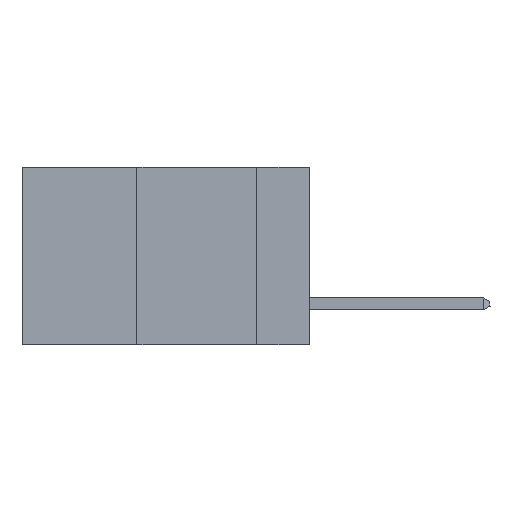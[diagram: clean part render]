
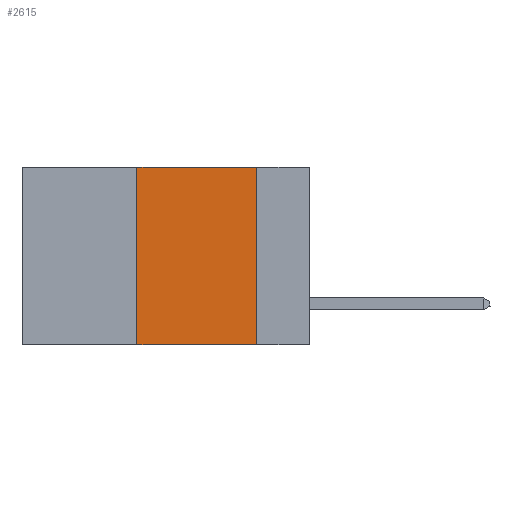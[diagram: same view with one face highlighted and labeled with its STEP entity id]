
A CAD part, left-side view. The second image highlights one B-rep face of the part: STEP entity #2615.
In plain terms, the highlighted planar face has unit normal (-1, 0, 0).
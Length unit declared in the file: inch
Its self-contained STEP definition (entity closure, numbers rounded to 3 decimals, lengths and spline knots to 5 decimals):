
#247 = CARTESIAN_POINT ( 'NONE',  ( 0., 0.11, -0.37 ) ) ;
#796 = CARTESIAN_POINT ( 'NONE',  ( 0., 0.6, 0. ) ) ;
#1013 = VECTOR ( 'NONE', #9403, 39.37008 ) ;
#1615 = EDGE_CURVE ( 'NONE', #12031, #11859, #6972, .T. ) ;
#2241 = DIRECTION ( 'NONE',  ( 0., 0., -1. ) ) ;
#2468 = AXIS2_PLACEMENT_3D ( 'NONE', #796, #4886, #2241 ) ;
#2615 = ADVANCED_FACE ( 'NONE', ( #13251 ), #14352, .F. ) ;
#3099 = LINE ( 'NONE', #13943, #3928 ) ;
#3928 = VECTOR ( 'NONE', #15187, 39.37008 ) ;
#4886 = DIRECTION ( 'NONE',  ( 1., 0., 0. ) ) ;
#5456 = VERTEX_POINT ( 'NONE', #12373 ) ;
#5460 = EDGE_CURVE ( 'NONE', #12031, #5456, #16967, .T. ) ;
#6972 = LINE ( 'NONE', #14789, #1013 ) ;
#7619 = ORIENTED_EDGE ( 'NONE', *, *, #5460, .F. ) ;
#8349 = CARTESIAN_POINT ( 'NONE',  ( 0., 0.36, 0. ) ) ;
#9403 = DIRECTION ( 'NONE',  ( 0., -1., 0. ) ) ;
#10386 = CARTESIAN_POINT ( 'NONE',  ( 0., 0.36, -0.37 ) ) ;
#10608 = VECTOR ( 'NONE', #14988, 39.37008 ) ;
#11859 = VERTEX_POINT ( 'NONE', #247 ) ;
#12031 = VERTEX_POINT ( 'NONE', #10386 ) ;
#12373 = CARTESIAN_POINT ( 'NONE',  ( 0., 0.36, 0. ) ) ;
#13206 = ORIENTED_EDGE ( 'NONE', *, *, #1615, .T. ) ;
#13251 = FACE_OUTER_BOUND ( 'NONE', #14702, .T. ) ;
#13943 = CARTESIAN_POINT ( 'NONE',  ( 0., 0.11, 0. ) ) ;
#14039 = ORIENTED_EDGE ( 'NONE', *, *, #15873, .F. ) ;
#14069 = CARTESIAN_POINT ( 'NONE',  ( 0., 0.6, 0. ) ) ;
#14299 = DIRECTION ( 'NONE',  ( 0., -1., 0. ) ) ;
#14352 = PLANE ( 'NONE',  #2468 ) ;
#14528 = LINE ( 'NONE', #14069, #16883 ) ;
#14702 = EDGE_LOOP ( 'NONE', ( #14039, #16604, #7619, #13206 ) ) ;
#14789 = CARTESIAN_POINT ( 'NONE',  ( 0., 0.6, -0.37 ) ) ;
#14988 = DIRECTION ( 'NONE',  ( 0., 0., 1. ) ) ;
#15106 = CARTESIAN_POINT ( 'NONE',  ( 0., 0.11, 0. ) ) ;
#15187 = DIRECTION ( 'NONE',  ( 0., 0., -1. ) ) ;
#15440 = EDGE_CURVE ( 'NONE', #5456, #16450, #14528, .T. ) ;
#15873 = EDGE_CURVE ( 'NONE', #16450, #11859, #3099, .T. ) ;
#16450 = VERTEX_POINT ( 'NONE', #15106 ) ;
#16604 = ORIENTED_EDGE ( 'NONE', *, *, #15440, .F. ) ;
#16883 = VECTOR ( 'NONE', #14299, 39.37008 ) ;
#16967 = LINE ( 'NONE', #8349, #10608 ) ;
